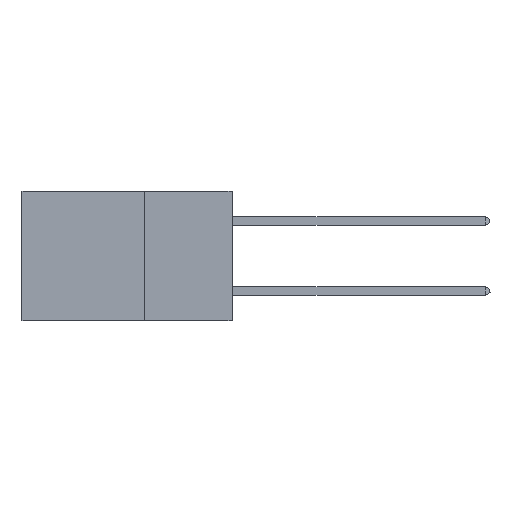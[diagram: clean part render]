
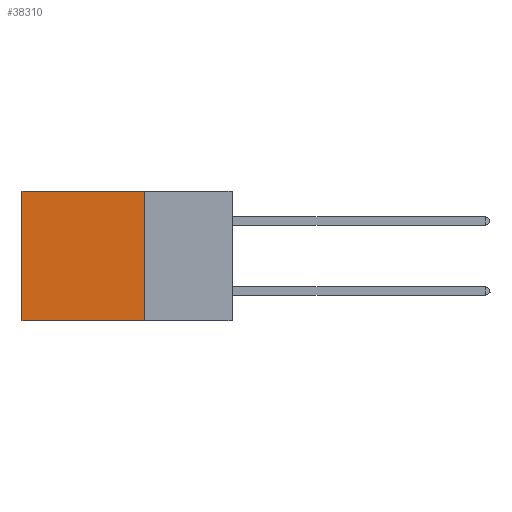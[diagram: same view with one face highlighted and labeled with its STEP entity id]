
A CAD part, left-side view. The second image highlights one B-rep face of the part: STEP entity #38310.
In plain terms, the highlighted planar face has unit normal (-1, 0, 0).
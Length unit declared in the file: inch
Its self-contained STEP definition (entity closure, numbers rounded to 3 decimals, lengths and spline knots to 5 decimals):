
#161 = CARTESIAN_POINT ( 'NONE',  ( 0.2875, 0.6, 0. ) ) ;
#617 = FACE_OUTER_BOUND ( 'NONE', #44066, .T. ) ;
#3992 = DIRECTION ( 'NONE',  ( 1., 0., 0. ) ) ;
#4699 = EDGE_CURVE ( 'NONE', #35269, #43404, #6347, .T. ) ;
#5738 = LINE ( 'NONE', #32086, #22799 ) ;
#6347 = LINE ( 'NONE', #7012, #13593 ) ;
#7012 = CARTESIAN_POINT ( 'NONE',  ( 0.2875, 0.6, 0. ) ) ;
#7426 = CARTESIAN_POINT ( 'NONE',  ( 0.2875, 0.6, -0.37 ) ) ;
#8219 = DIRECTION ( 'NONE',  ( 0., 1., 0. ) ) ;
#11179 = DIRECTION ( 'NONE',  ( 0., 0., -1. ) ) ;
#11746 = LINE ( 'NONE', #25487, #19746 ) ;
#12444 = CARTESIAN_POINT ( 'NONE',  ( 0.2875, 0.25, 0. ) ) ;
#13593 = VECTOR ( 'NONE', #13773, 39.37008 ) ;
#13773 = DIRECTION ( 'NONE',  ( 0., 0., -1. ) ) ;
#13912 = PLANE ( 'NONE',  #22452 ) ;
#14313 = VECTOR ( 'NONE', #36954, 39.37008 ) ;
#16593 = CARTESIAN_POINT ( 'NONE',  ( 0.2875, 0.25, -0.37 ) ) ;
#17272 = EDGE_CURVE ( 'NONE', #35267, #43404, #11746, .T. ) ;
#17611 = ORIENTED_EDGE ( 'NONE', *, *, #41924, .F. ) ;
#19746 = VECTOR ( 'NONE', #39211, 39.37008 ) ;
#19994 = EDGE_CURVE ( 'NONE', #31823, #35269, #5738, .T. ) ;
#21767 = ORIENTED_EDGE ( 'NONE', *, *, #19994, .T. ) ;
#22452 = AXIS2_PLACEMENT_3D ( 'NONE', #34859, #3992, #11179 ) ;
#22799 = VECTOR ( 'NONE', #8219, 39.37008 ) ;
#24138 = ORIENTED_EDGE ( 'NONE', *, *, #17272, .F. ) ;
#25487 = CARTESIAN_POINT ( 'NONE',  ( 0.2875, 0.25, -0.37 ) ) ;
#28940 = ORIENTED_EDGE ( 'NONE', *, *, #4699, .T. ) ;
#31823 = VERTEX_POINT ( 'NONE', #12444 ) ;
#32086 = CARTESIAN_POINT ( 'NONE',  ( 0.2875, 0.25, 0. ) ) ;
#33799 = LINE ( 'NONE', #40319, #14313 ) ;
#34859 = CARTESIAN_POINT ( 'NONE',  ( 0.2875, 0.25, 0. ) ) ;
#35267 = VERTEX_POINT ( 'NONE', #16593 ) ;
#35269 = VERTEX_POINT ( 'NONE', #161 ) ;
#36954 = DIRECTION ( 'NONE',  ( 0., 0., -1. ) ) ;
#38310 = ADVANCED_FACE ( 'NONE', ( #617 ), #13912, .F. ) ;
#39211 = DIRECTION ( 'NONE',  ( 0., 1., 0. ) ) ;
#40319 = CARTESIAN_POINT ( 'NONE',  ( 0.2875, 0.25, 0. ) ) ;
#41924 = EDGE_CURVE ( 'NONE', #31823, #35267, #33799, .T. ) ;
#43404 = VERTEX_POINT ( 'NONE', #7426 ) ;
#44066 = EDGE_LOOP ( 'NONE', ( #28940, #24138, #17611, #21767 ) ) ;
